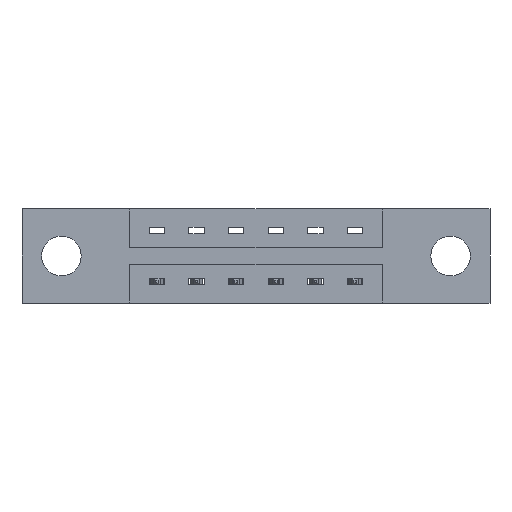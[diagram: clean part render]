
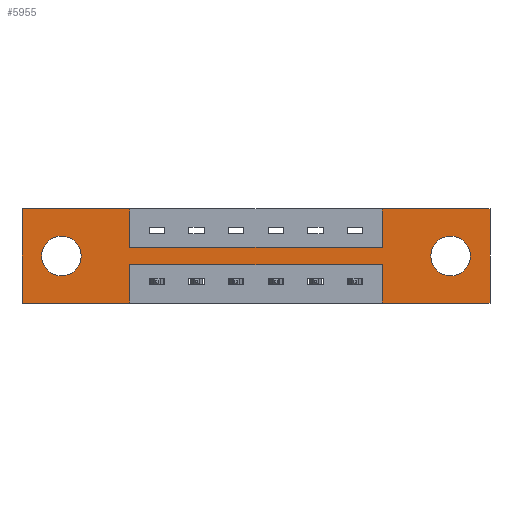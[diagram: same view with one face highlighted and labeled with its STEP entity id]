
A CAD part, front view. The second image highlights one B-rep face of the part: STEP entity #5955.
In plain terms, the highlighted planar face has unit normal (0, -1, 0).
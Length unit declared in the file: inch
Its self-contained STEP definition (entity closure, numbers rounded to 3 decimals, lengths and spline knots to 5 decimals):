
#1 = VERTEX_POINT ( 'NONE', #6184 ) ;
#61 = CARTESIAN_POINT ( 'NONE',  ( 0., 0., 0. ) ) ;
#218 = EDGE_CURVE ( 'NONE', #6256, #7365, #4054, .T. ) ;
#310 = DIRECTION ( 'NONE',  ( 0., 1., 0. ) ) ;
#352 = VECTOR ( 'NONE', #8440, 39.37008 ) ;
#369 = CARTESIAN_POINT ( 'NONE',  ( 1.417, 0., -0.37 ) ) ;
#385 = VERTEX_POINT ( 'NONE', #1027 ) ;
#518 = VECTOR ( 'NONE', #7622, 39.37008 ) ;
#641 = CARTESIAN_POINT ( 'NONE',  ( 0.425, 0., -0.22 ) ) ;
#650 = DIRECTION ( 'NONE',  ( 0., 0., -1. ) ) ;
#741 = ORIENTED_EDGE ( 'NONE', *, *, #5351, .F. ) ;
#747 = PLANE ( 'NONE',  #2109 ) ;
#754 = LINE ( 'NONE', #61, #518 ) ;
#822 = CIRCLE ( 'NONE', #895, 0.078 ) ;
#873 = AXIS2_PLACEMENT_3D ( 'NONE', #8687, #310, #6128 ) ;
#890 = VERTEX_POINT ( 'NONE', #8903 ) ;
#895 = AXIS2_PLACEMENT_3D ( 'NONE', #6098, #1864, #6781 ) ;
#967 = VERTEX_POINT ( 'NONE', #7693 ) ;
#988 = ORIENTED_EDGE ( 'NONE', *, *, #7709, .F. ) ;
#1020 = LINE ( 'NONE', #3367, #6480 ) ;
#1027 = CARTESIAN_POINT ( 'NONE',  ( 1.842, 0., -0.37 ) ) ;
#1036 = CIRCLE ( 'NONE', #2025, 0.078 ) ;
#1076 = EDGE_CURVE ( 'NONE', #5711, #1273, #8446, .T. ) ;
#1150 = CARTESIAN_POINT ( 'NONE',  ( 0.425, 0., -0.15 ) ) ;
#1273 = VERTEX_POINT ( 'NONE', #7880 ) ;
#1347 = VECTOR ( 'NONE', #6156, 39.37008 ) ;
#1350 = VERTEX_POINT ( 'NONE', #8527 ) ;
#1422 = CARTESIAN_POINT ( 'NONE',  ( 1.687, 0., -0.107 ) ) ;
#1431 = DIRECTION ( 'NONE',  ( 0., 0., -1. ) ) ;
#1433 = FACE_BOUND ( 'NONE', #6370, .T. ) ;
#1531 = ORIENTED_EDGE ( 'NONE', *, *, #3730, .F. ) ;
#1537 = DIRECTION ( 'NONE',  ( 0., 0., 1. ) ) ;
#1624 = EDGE_CURVE ( 'NONE', #2192, #967, #8060, .T. ) ;
#1812 = EDGE_CURVE ( 'NONE', #7699, #3492, #1036, .T. ) ;
#1864 = DIRECTION ( 'NONE',  ( 0., 1., 0. ) ) ;
#1977 = VECTOR ( 'NONE', #1431, 39.37008 ) ;
#1992 = ORIENTED_EDGE ( 'NONE', *, *, #6901, .F. ) ;
#2023 = VECTOR ( 'NONE', #5528, 39.37008 ) ;
#2025 = AXIS2_PLACEMENT_3D ( 'NONE', #4154, #7921, #8432 ) ;
#2100 = DIRECTION ( 'NONE',  ( 0., 0., 1. ) ) ;
#2109 = AXIS2_PLACEMENT_3D ( 'NONE', #3708, #6487, #2285 ) ;
#2168 = CARTESIAN_POINT ( 'NONE',  ( 0.425, 0., -0.37 ) ) ;
#2192 = VERTEX_POINT ( 'NONE', #4662 ) ;
#2285 = DIRECTION ( 'NONE',  ( 0., 0., -1. ) ) ;
#2382 = LINE ( 'NONE', #6396, #5893 ) ;
#2596 = CARTESIAN_POINT ( 'NONE',  ( 1.687, 0., -0.263 ) ) ;
#2696 = VECTOR ( 'NONE', #3633, 39.37008 ) ;
#2779 = ORIENTED_EDGE ( 'NONE', *, *, #4497, .F. ) ;
#2937 = AXIS2_PLACEMENT_3D ( 'NONE', #8891, #8925, #8969 ) ;
#3101 = LINE ( 'NONE', #1150, #1347 ) ;
#3143 = ORIENTED_EDGE ( 'NONE', *, *, #3547, .F. ) ;
#3243 = CARTESIAN_POINT ( 'NONE',  ( 0., 0., -0.37 ) ) ;
#3250 = EDGE_CURVE ( 'NONE', #1273, #1350, #754, .T. ) ;
#3367 = CARTESIAN_POINT ( 'NONE',  ( 0., 0., -0.37 ) ) ;
#3373 = CARTESIAN_POINT ( 'NONE',  ( 1.417, 0., -0.37 ) ) ;
#3400 = EDGE_LOOP ( 'NONE', ( #8870, #3143, #1992, #7202, #1531, #7418, #6621, #2779, #6866, #6442, #741, #988 ) ) ;
#3428 = ORIENTED_EDGE ( 'NONE', *, *, #3758, .T. ) ;
#3484 = CARTESIAN_POINT ( 'NONE',  ( 1.417, 0., -0.22 ) ) ;
#3492 = VERTEX_POINT ( 'NONE', #1422 ) ;
#3547 = EDGE_CURVE ( 'NONE', #5740, #8539, #5336, .T. ) ;
#3633 = DIRECTION ( 'NONE',  ( 1., 0., 0. ) ) ;
#3663 = CARTESIAN_POINT ( 'NONE',  ( 0.155, 0., -0.263 ) ) ;
#3674 = CIRCLE ( 'NONE', #873, 0.078 ) ;
#3708 = CARTESIAN_POINT ( 'NONE',  ( 0., 0., -0.37 ) ) ;
#3730 = EDGE_CURVE ( 'NONE', #1350, #385, #6167, .T. ) ;
#3758 = EDGE_CURVE ( 'NONE', #7365, #6256, #3674, .T. ) ;
#3853 = ORIENTED_EDGE ( 'NONE', *, *, #6212, .T. ) ;
#3889 = LINE ( 'NONE', #3243, #7376 ) ;
#3931 = LINE ( 'NONE', #3373, #2023 ) ;
#3999 = VERTEX_POINT ( 'NONE', #369 ) ;
#4042 = CARTESIAN_POINT ( 'NONE',  ( 0.425, 0., -0.22 ) ) ;
#4054 = CIRCLE ( 'NONE', #2937, 0.078 ) ;
#4154 = CARTESIAN_POINT ( 'NONE',  ( 1.687, 0., -0.185 ) ) ;
#4257 = VERTEX_POINT ( 'NONE', #7279 ) ;
#4497 = EDGE_CURVE ( 'NONE', #1, #5711, #3101, .T. ) ;
#4662 = CARTESIAN_POINT ( 'NONE',  ( 0., 0., 0. ) ) ;
#5067 = ORIENTED_EDGE ( 'NONE', *, *, #1812, .T. ) ;
#5150 = CARTESIAN_POINT ( 'NONE',  ( 0., 0., 0. ) ) ;
#5336 = LINE ( 'NONE', #4042, #7112 ) ;
#5351 = EDGE_CURVE ( 'NONE', #4257, #2192, #8982, .T. ) ;
#5420 = VECTOR ( 'NONE', #1537, 39.37008 ) ;
#5528 = DIRECTION ( 'NONE',  ( 0., 0., 1. ) ) ;
#5579 = CARTESIAN_POINT ( 'NONE',  ( 1.417, 0., -0.15 ) ) ;
#5711 = VERTEX_POINT ( 'NONE', #5579 ) ;
#5740 = VERTEX_POINT ( 'NONE', #3484 ) ;
#5865 = EDGE_CURVE ( 'NONE', #8539, #890, #6760, .T. ) ;
#5875 = EDGE_CURVE ( 'NONE', #967, #1, #2382, .T. ) ;
#5893 = VECTOR ( 'NONE', #650, 39.37008 ) ;
#5955 = ADVANCED_FACE ( 'NONE', ( #7077, #1433, #8876 ), #747, .T. ) ;
#6090 = CARTESIAN_POINT ( 'NONE',  ( 0., 0., 0. ) ) ;
#6098 = CARTESIAN_POINT ( 'NONE',  ( 1.687, 0., -0.185 ) ) ;
#6128 = DIRECTION ( 'NONE',  ( 0., 0., 1. ) ) ;
#6156 = DIRECTION ( 'NONE',  ( 1., 0., 0. ) ) ;
#6167 = LINE ( 'NONE', #9154, #1977 ) ;
#6184 = CARTESIAN_POINT ( 'NONE',  ( 0.425, 0., -0.15 ) ) ;
#6212 = EDGE_CURVE ( 'NONE', #3492, #7699, #822, .T. ) ;
#6256 = VERTEX_POINT ( 'NONE', #7550 ) ;
#6370 = EDGE_LOOP ( 'NONE', ( #8567, #3428 ) ) ;
#6396 = CARTESIAN_POINT ( 'NONE',  ( 0.425, 0., 0. ) ) ;
#6402 = VECTOR ( 'NONE', #2100, 39.37008 ) ;
#6442 = ORIENTED_EDGE ( 'NONE', *, *, #1624, .F. ) ;
#6480 = VECTOR ( 'NONE', #8218, 39.37008 ) ;
#6487 = DIRECTION ( 'NONE',  ( 0., -1., 0. ) ) ;
#6621 = ORIENTED_EDGE ( 'NONE', *, *, #1076, .F. ) ;
#6760 = LINE ( 'NONE', #2168, #352 ) ;
#6781 = DIRECTION ( 'NONE',  ( 0., 0., -1. ) ) ;
#6866 = ORIENTED_EDGE ( 'NONE', *, *, #5875, .F. ) ;
#6901 = EDGE_CURVE ( 'NONE', #3999, #5740, #3931, .T. ) ;
#7077 = FACE_BOUND ( 'NONE', #7356, .T. ) ;
#7112 = VECTOR ( 'NONE', #7650, 39.37008 ) ;
#7202 = ORIENTED_EDGE ( 'NONE', *, *, #7603, .F. ) ;
#7279 = CARTESIAN_POINT ( 'NONE',  ( 0., 0., -0.37 ) ) ;
#7356 = EDGE_LOOP ( 'NONE', ( #3853, #5067 ) ) ;
#7365 = VERTEX_POINT ( 'NONE', #3663 ) ;
#7376 = VECTOR ( 'NONE', #8102, 39.37008 ) ;
#7418 = ORIENTED_EDGE ( 'NONE', *, *, #3250, .F. ) ;
#7550 = CARTESIAN_POINT ( 'NONE',  ( 0.155, 0., -0.107 ) ) ;
#7603 = EDGE_CURVE ( 'NONE', #385, #3999, #3889, .T. ) ;
#7622 = DIRECTION ( 'NONE',  ( 1., 0., 0. ) ) ;
#7650 = DIRECTION ( 'NONE',  ( -1., 0., 0. ) ) ;
#7693 = CARTESIAN_POINT ( 'NONE',  ( 0.425, 0., 0. ) ) ;
#7699 = VERTEX_POINT ( 'NONE', #2596 ) ;
#7709 = EDGE_CURVE ( 'NONE', #890, #4257, #1020, .T. ) ;
#7880 = CARTESIAN_POINT ( 'NONE',  ( 1.417, 0., 0. ) ) ;
#7921 = DIRECTION ( 'NONE',  ( 0., 1., 0. ) ) ;
#8060 = LINE ( 'NONE', #6090, #2696 ) ;
#8102 = DIRECTION ( 'NONE',  ( -1., 0., 0. ) ) ;
#8218 = DIRECTION ( 'NONE',  ( -1., 0., 0. ) ) ;
#8432 = DIRECTION ( 'NONE',  ( 0., 0., -1. ) ) ;
#8440 = DIRECTION ( 'NONE',  ( 0., 0., -1. ) ) ;
#8446 = LINE ( 'NONE', #8598, #6402 ) ;
#8527 = CARTESIAN_POINT ( 'NONE',  ( 1.842, 0., 0. ) ) ;
#8539 = VERTEX_POINT ( 'NONE', #641 ) ;
#8567 = ORIENTED_EDGE ( 'NONE', *, *, #218, .T. ) ;
#8598 = CARTESIAN_POINT ( 'NONE',  ( 1.417, 0., 0. ) ) ;
#8687 = CARTESIAN_POINT ( 'NONE',  ( 0.155, 0., -0.185 ) ) ;
#8870 = ORIENTED_EDGE ( 'NONE', *, *, #5865, .F. ) ;
#8876 = FACE_OUTER_BOUND ( 'NONE', #3400, .T. ) ;
#8891 = CARTESIAN_POINT ( 'NONE',  ( 0.155, 0., -0.185 ) ) ;
#8903 = CARTESIAN_POINT ( 'NONE',  ( 0.425, 0., -0.37 ) ) ;
#8925 = DIRECTION ( 'NONE',  ( 0., 1., 0. ) ) ;
#8969 = DIRECTION ( 'NONE',  ( 0., 0., 1. ) ) ;
#8982 = LINE ( 'NONE', #5150, #5420 ) ;
#9154 = CARTESIAN_POINT ( 'NONE',  ( 1.842, 0., 0. ) ) ;
